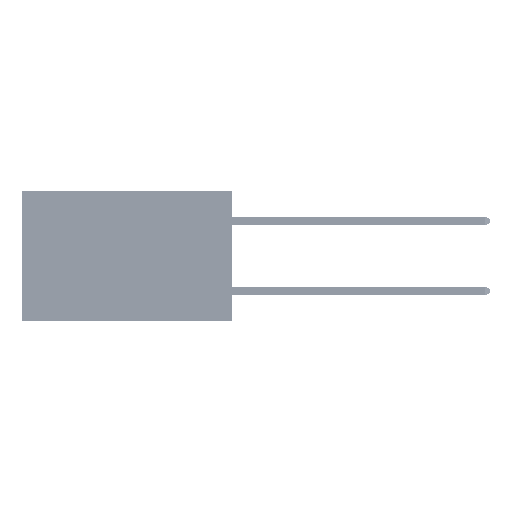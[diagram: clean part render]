
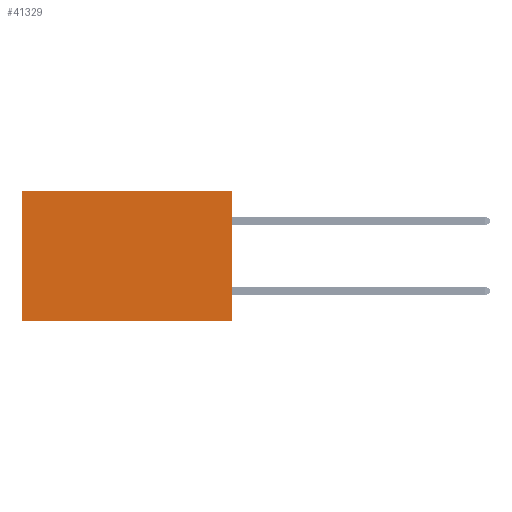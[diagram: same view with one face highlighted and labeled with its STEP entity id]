
A CAD part, left-side view. The second image highlights one B-rep face of the part: STEP entity #41329.
In plain terms, the highlighted planar face has unit normal (-1, 0, 0).
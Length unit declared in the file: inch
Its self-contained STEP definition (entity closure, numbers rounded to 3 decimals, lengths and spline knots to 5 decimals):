
#311 = CARTESIAN_POINT ( 'NONE',  ( 0.2875, 0., 0. ) ) ;
#3965 = EDGE_CURVE ( 'NONE', #17335, #36796, #16569, .T. ) ;
#4392 = DIRECTION ( 'NONE',  ( 0., 0., -1. ) ) ;
#7482 = LINE ( 'NONE', #33019, #15648 ) ;
#7558 = DIRECTION ( 'NONE',  ( 0., 0., -1. ) ) ;
#7847 = FACE_OUTER_BOUND ( 'NONE', #42483, .T. ) ;
#8046 = DIRECTION ( 'NONE',  ( 0., 0., -1. ) ) ;
#9281 = CARTESIAN_POINT ( 'NONE',  ( 0.2875, 0., -0.37 ) ) ;
#10832 = LINE ( 'NONE', #31420, #35569 ) ;
#15531 = DIRECTION ( 'NONE',  ( 0., 1., 0. ) ) ;
#15648 = VECTOR ( 'NONE', #44797, 39.37008 ) ;
#16569 = LINE ( 'NONE', #46676, #37470 ) ;
#17335 = VERTEX_POINT ( 'NONE', #31862 ) ;
#19508 = ORIENTED_EDGE ( 'NONE', *, *, #21478, .F. ) ;
#20140 = CARTESIAN_POINT ( 'NONE',  ( 0.2875, 0., 0. ) ) ;
#21478 = EDGE_CURVE ( 'NONE', #42029, #36796, #10832, .T. ) ;
#22490 = ORIENTED_EDGE ( 'NONE', *, *, #3965, .T. ) ;
#24298 = PLANE ( 'NONE',  #46417 ) ;
#26000 = LINE ( 'NONE', #20140, #45407 ) ;
#28273 = DIRECTION ( 'NONE',  ( 1., 0., 0. ) ) ;
#29302 = ORIENTED_EDGE ( 'NONE', *, *, #45094, .T. ) ;
#31420 = CARTESIAN_POINT ( 'NONE',  ( 0.2875, 0., -0.37 ) ) ;
#31862 = CARTESIAN_POINT ( 'NONE',  ( 0.2875, 0.6, 0. ) ) ;
#33019 = CARTESIAN_POINT ( 'NONE',  ( 0.2875, 0., 0. ) ) ;
#33308 = VERTEX_POINT ( 'NONE', #48110 ) ;
#35569 = VECTOR ( 'NONE', #15531, 39.37008 ) ;
#36796 = VERTEX_POINT ( 'NONE', #45347 ) ;
#37470 = VECTOR ( 'NONE', #7558, 39.37008 ) ;
#37919 = ORIENTED_EDGE ( 'NONE', *, *, #46801, .F. ) ;
#41329 = ADVANCED_FACE ( 'NONE', ( #7847 ), #24298, .F. ) ;
#42029 = VERTEX_POINT ( 'NONE', #9281 ) ;
#42483 = EDGE_LOOP ( 'NONE', ( #22490, #19508, #37919, #29302 ) ) ;
#44797 = DIRECTION ( 'NONE',  ( 0., 1., 0. ) ) ;
#45094 = EDGE_CURVE ( 'NONE', #33308, #17335, #7482, .T. ) ;
#45347 = CARTESIAN_POINT ( 'NONE',  ( 0.2875, 0.6, -0.37 ) ) ;
#45407 = VECTOR ( 'NONE', #8046, 39.37008 ) ;
#46417 = AXIS2_PLACEMENT_3D ( 'NONE', #311, #28273, #4392 ) ;
#46676 = CARTESIAN_POINT ( 'NONE',  ( 0.2875, 0.6, 0. ) ) ;
#46801 = EDGE_CURVE ( 'NONE', #33308, #42029, #26000, .T. ) ;
#48110 = CARTESIAN_POINT ( 'NONE',  ( 0.2875, 0., 0. ) ) ;
